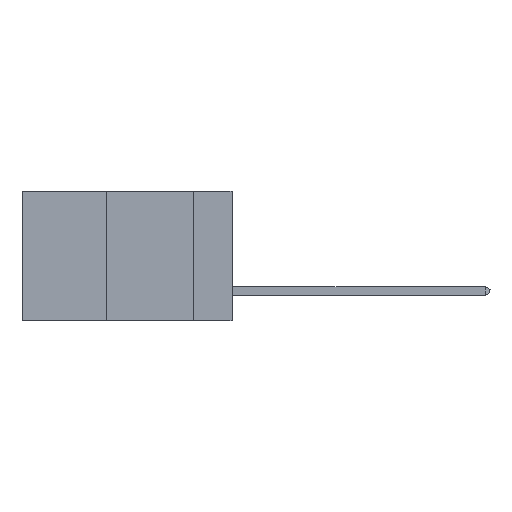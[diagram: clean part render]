
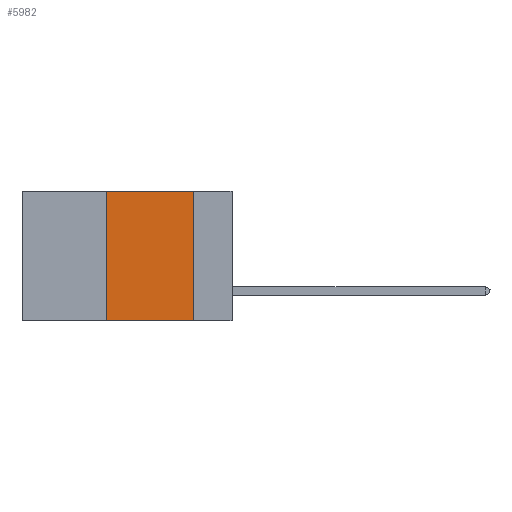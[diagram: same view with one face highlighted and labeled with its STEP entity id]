
A CAD part, left-side view. The second image highlights one B-rep face of the part: STEP entity #5982.
In plain terms, the highlighted planar face has unit normal (-1, 0, 0).
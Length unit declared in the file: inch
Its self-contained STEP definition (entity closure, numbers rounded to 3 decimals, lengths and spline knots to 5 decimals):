
#297 = VERTEX_POINT ( 'NONE', #1227 ) ;
#385 = ORIENTED_EDGE ( 'NONE', *, *, #4306, .F. ) ;
#765 = DIRECTION ( 'NONE',  ( 1., 0., 0. ) ) ;
#796 = EDGE_CURVE ( 'NONE', #10732, #8527, #25198, .T. ) ;
#1227 = CARTESIAN_POINT ( 'NONE',  ( 0., 0.36, 0. ) ) ;
#4306 = EDGE_CURVE ( 'NONE', #9889, #8527, #12030, .T. ) ;
#5239 = CARTESIAN_POINT ( 'NONE',  ( 0., 0.11, 0. ) ) ;
#5275 = CARTESIAN_POINT ( 'NONE',  ( 0., 0.36, -0.37 ) ) ;
#5781 = ORIENTED_EDGE ( 'NONE', *, *, #16674, .F. ) ;
#5982 = ADVANCED_FACE ( 'NONE', ( #10801 ), #27056, .F. ) ;
#7388 = ORIENTED_EDGE ( 'NONE', *, *, #15489, .F. ) ;
#8527 = VERTEX_POINT ( 'NONE', #18369 ) ;
#8802 = VECTOR ( 'NONE', #25584, 39.37008 ) ;
#9492 = VECTOR ( 'NONE', #12787, 39.37008 ) ;
#9889 = VERTEX_POINT ( 'NONE', #22022 ) ;
#10732 = VERTEX_POINT ( 'NONE', #5275 ) ;
#10801 = FACE_OUTER_BOUND ( 'NONE', #26591, .T. ) ;
#12030 = LINE ( 'NONE', #5239, #30358 ) ;
#12787 = DIRECTION ( 'NONE',  ( 0., 0., 1. ) ) ;
#14822 = ORIENTED_EDGE ( 'NONE', *, *, #796, .T. ) ;
#14947 = CARTESIAN_POINT ( 'NONE',  ( 0., 0.6, 0. ) ) ;
#15489 = EDGE_CURVE ( 'NONE', #10732, #297, #15825, .T. ) ;
#15825 = LINE ( 'NONE', #24784, #9492 ) ;
#16499 = VECTOR ( 'NONE', #25496, 39.37008 ) ;
#16674 = EDGE_CURVE ( 'NONE', #297, #9889, #17251, .T. ) ;
#17251 = LINE ( 'NONE', #30038, #16499 ) ;
#18369 = CARTESIAN_POINT ( 'NONE',  ( 0., 0.11, -0.37 ) ) ;
#21132 = CARTESIAN_POINT ( 'NONE',  ( 0., 0.6, -0.37 ) ) ;
#21897 = DIRECTION ( 'NONE',  ( 0., 0., -1. ) ) ;
#22022 = CARTESIAN_POINT ( 'NONE',  ( 0., 0.11, 0. ) ) ;
#24759 = DIRECTION ( 'NONE',  ( 0., 0., -1. ) ) ;
#24784 = CARTESIAN_POINT ( 'NONE',  ( 0., 0.36, 0. ) ) ;
#25198 = LINE ( 'NONE', #21132, #8802 ) ;
#25496 = DIRECTION ( 'NONE',  ( 0., -1., 0. ) ) ;
#25584 = DIRECTION ( 'NONE',  ( 0., -1., 0. ) ) ;
#26591 = EDGE_LOOP ( 'NONE', ( #385, #5781, #7388, #14822 ) ) ;
#27056 = PLANE ( 'NONE',  #30324 ) ;
#30038 = CARTESIAN_POINT ( 'NONE',  ( 0., 0.6, 0. ) ) ;
#30324 = AXIS2_PLACEMENT_3D ( 'NONE', #14947, #765, #24759 ) ;
#30358 = VECTOR ( 'NONE', #21897, 39.37008 ) ;
